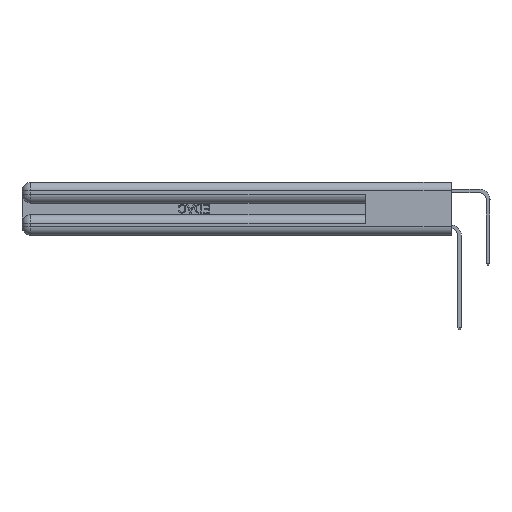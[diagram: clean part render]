
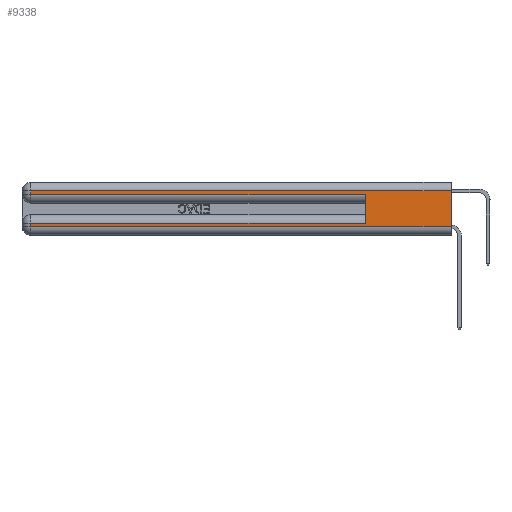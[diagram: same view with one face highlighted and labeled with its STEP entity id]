
A CAD part, left-side view. The second image highlights one B-rep face of the part: STEP entity #9338.
In plain terms, the highlighted planar face has unit normal (-1, 0, 0).
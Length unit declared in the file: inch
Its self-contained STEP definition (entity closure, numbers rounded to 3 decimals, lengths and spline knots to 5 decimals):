
#166 = ORIENTED_EDGE ( 'NONE', *, *, #5029, .T. ) ;
#803 = LINE ( 'NONE', #7151, #36604 ) ;
#1402 = ORIENTED_EDGE ( 'NONE', *, *, #19467, .T. ) ;
#1547 = CARTESIAN_POINT ( 'NONE',  ( 0., 0.6, 0.285 ) ) ;
#3018 = VERTEX_POINT ( 'NONE', #14544 ) ;
#3612 = VERTEX_POINT ( 'NONE', #6859 ) ;
#3956 = EDGE_CURVE ( 'NONE', #13253, #14883, #11842, .T. ) ;
#4874 = LINE ( 'NONE', #30860, #34779 ) ;
#5029 = EDGE_CURVE ( 'NONE', #3018, #21477, #5367, .T. ) ;
#5367 = LINE ( 'NONE', #6715, #8553 ) ;
#5526 = VERTEX_POINT ( 'NONE', #13261 ) ;
#5717 = DIRECTION ( 'NONE',  ( 0., 0., -1. ) ) ;
#5918 = EDGE_CURVE ( 'NONE', #21477, #14883, #16644, .T. ) ;
#6715 = CARTESIAN_POINT ( 'NONE',  ( 0., 2.94, 0.37 ) ) ;
#6859 = CARTESIAN_POINT ( 'NONE',  ( 0., 2.94, 0.085 ) ) ;
#7151 = CARTESIAN_POINT ( 'NONE',  ( 0., 0., 0.06 ) ) ;
#7477 = ORIENTED_EDGE ( 'NONE', *, *, #8134, .F. ) ;
#7765 = VERTEX_POINT ( 'NONE', #21158 ) ;
#7858 = VECTOR ( 'NONE', #17923, 39.37008 ) ;
#8134 = EDGE_CURVE ( 'NONE', #7765, #5526, #11737, .T. ) ;
#8553 = VECTOR ( 'NONE', #26490, 39.37008 ) ;
#8629 = EDGE_CURVE ( 'NONE', #3612, #24925, #4874, .T. ) ;
#9338 = ADVANCED_FACE ( 'NONE', ( #27480 ), #37516, .F. ) ;
#10495 = AXIS2_PLACEMENT_3D ( 'NONE', #23074, #34983, #5717 ) ;
#11670 = CARTESIAN_POINT ( 'NONE',  ( 0., 0., 0.31 ) ) ;
#11737 = LINE ( 'NONE', #27016, #33008 ) ;
#11842 = LINE ( 'NONE', #33780, #36277 ) ;
#13253 = VERTEX_POINT ( 'NONE', #28654 ) ;
#13261 = CARTESIAN_POINT ( 'NONE',  ( 0., 0., 0.06 ) ) ;
#14544 = CARTESIAN_POINT ( 'NONE',  ( 0., 2.94, 0.31 ) ) ;
#14883 = VERTEX_POINT ( 'NONE', #1547 ) ;
#16289 = ORIENTED_EDGE ( 'NONE', *, *, #26405, .T. ) ;
#16644 = LINE ( 'NONE', #20308, #31664 ) ;
#17923 = DIRECTION ( 'NONE',  ( 0., 1., 0. ) ) ;
#18002 = DIRECTION ( 'NONE',  ( 0., 0., -1. ) ) ;
#19467 = EDGE_CURVE ( 'NONE', #24925, #5526, #803, .T. ) ;
#19488 = EDGE_LOOP ( 'NONE', ( #7477, #16289, #166, #30072, #27915, #26561, #25754, #1402 ) ) ;
#20308 = CARTESIAN_POINT ( 'NONE',  ( 0., 0., 0.285 ) ) ;
#20840 = CARTESIAN_POINT ( 'NONE',  ( 0., 0., 0.085 ) ) ;
#20983 = EDGE_CURVE ( 'NONE', #13253, #3612, #28742, .T. ) ;
#21158 = CARTESIAN_POINT ( 'NONE',  ( 0., 0., 0.31 ) ) ;
#21477 = VERTEX_POINT ( 'NONE', #37404 ) ;
#22409 = VECTOR ( 'NONE', #31820, 39.37008 ) ;
#23074 = CARTESIAN_POINT ( 'NONE',  ( 0., 0., 0.37 ) ) ;
#24925 = VERTEX_POINT ( 'NONE', #28598 ) ;
#25116 = LINE ( 'NONE', #11670, #22409 ) ;
#25661 = DIRECTION ( 'NONE',  ( 0., 0., 1. ) ) ;
#25754 = ORIENTED_EDGE ( 'NONE', *, *, #8629, .T. ) ;
#26405 = EDGE_CURVE ( 'NONE', #7765, #3018, #25116, .T. ) ;
#26490 = DIRECTION ( 'NONE',  ( 0., 0., -1. ) ) ;
#26561 = ORIENTED_EDGE ( 'NONE', *, *, #20983, .T. ) ;
#27016 = CARTESIAN_POINT ( 'NONE',  ( 0., 0., 0.37 ) ) ;
#27480 = FACE_OUTER_BOUND ( 'NONE', #19488, .T. ) ;
#27915 = ORIENTED_EDGE ( 'NONE', *, *, #3956, .F. ) ;
#28598 = CARTESIAN_POINT ( 'NONE',  ( 0., 2.94, 0.06 ) ) ;
#28654 = CARTESIAN_POINT ( 'NONE',  ( 0., 0.6, 0.085 ) ) ;
#28742 = LINE ( 'NONE', #20840, #7858 ) ;
#29947 = DIRECTION ( 'NONE',  ( 0., 0., -1. ) ) ;
#30072 = ORIENTED_EDGE ( 'NONE', *, *, #5918, .T. ) ;
#30618 = DIRECTION ( 'NONE',  ( 0., -1., 0. ) ) ;
#30860 = CARTESIAN_POINT ( 'NONE',  ( 0., 2.94, 0.37 ) ) ;
#31664 = VECTOR ( 'NONE', #32232, 39.37008 ) ;
#31820 = DIRECTION ( 'NONE',  ( 0., 1., 0. ) ) ;
#32232 = DIRECTION ( 'NONE',  ( 0., -1., 0. ) ) ;
#33008 = VECTOR ( 'NONE', #29947, 39.37008 ) ;
#33780 = CARTESIAN_POINT ( 'NONE',  ( 0., 0.6, 0.145 ) ) ;
#34779 = VECTOR ( 'NONE', #18002, 39.37008 ) ;
#34983 = DIRECTION ( 'NONE',  ( 1., 0., 0. ) ) ;
#36277 = VECTOR ( 'NONE', #25661, 39.37008 ) ;
#36604 = VECTOR ( 'NONE', #30618, 39.37008 ) ;
#37404 = CARTESIAN_POINT ( 'NONE',  ( 0., 2.94, 0.285 ) ) ;
#37516 = PLANE ( 'NONE',  #10495 ) ;
